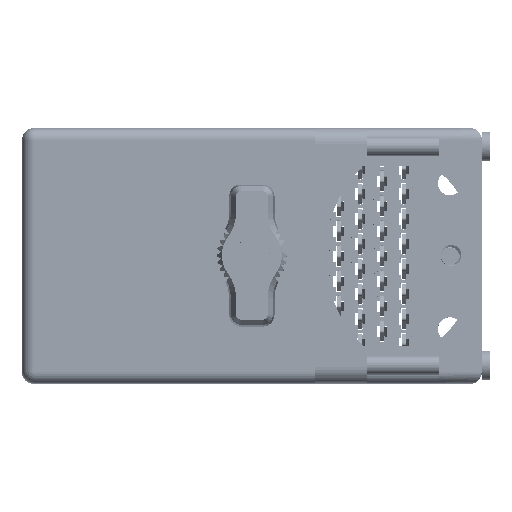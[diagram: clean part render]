
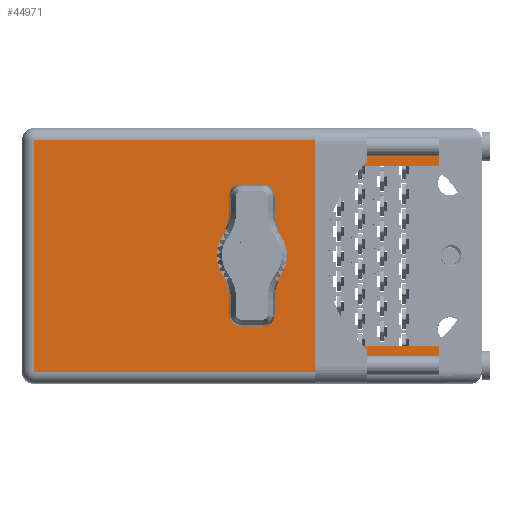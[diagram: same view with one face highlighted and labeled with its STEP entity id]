
A CAD part, top view. The second image highlights one B-rep face of the part: STEP entity #44971.
In plain terms, the highlighted face is planar.
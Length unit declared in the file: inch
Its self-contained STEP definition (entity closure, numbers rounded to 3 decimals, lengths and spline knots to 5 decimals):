
#1063 = DIRECTION ( 'NONE',  ( 0., 1., 0. ) ) ;
#3258 = AXIS2_PLACEMENT_3D ( 'NONE', #57674, #67712, #58091 ) ;
#4611 = CARTESIAN_POINT ( 'NONE',  ( 2.499, 2.03, -0.07 ) ) ;
#10472 = EDGE_CURVE ( 'NONE', #17656, #46219, #93250, .T. ) ;
#11401 = CARTESIAN_POINT ( 'NONE',  ( 1.3775, 2.03, -0.935 ) ) ;
#11614 = CARTESIAN_POINT ( 'NONE',  ( 2.499, 2.03, -1.305 ) ) ;
#12439 = ORIENTED_EDGE ( 'NONE', *, *, #10472, .F. ) ;
#12688 = CARTESIAN_POINT ( 'NONE',  ( 1.785, 2.03, -1.305 ) ) ;
#13154 = LINE ( 'NONE', #12688, #102062 ) ;
#13281 = LINE ( 'NONE', #101350, #80673 ) ;
#14627 = LINE ( 'NONE', #4611, #59185 ) ;
#15113 = CARTESIAN_POINT ( 'NONE',  ( 1.3775, 2.03, -0.595 ) ) ;
#15484 = VECTOR ( 'NONE', #58173, 39.37008 ) ;
#16676 = CIRCLE ( 'NONE', #3258, 0.17 ) ;
#17132 = EDGE_CURVE ( 'NONE', #26640, #64895, #16676, .T. ) ;
#17282 = VECTOR ( 'NONE', #108263, 39.37008 ) ;
#17656 = VERTEX_POINT ( 'NONE', #29456 ) ;
#19880 = ORIENTED_EDGE ( 'NONE', *, *, #88196, .T. ) ;
#20483 = EDGE_CURVE ( 'NONE', #95439, #37082, #14627, .T. ) ;
#22983 = VERTEX_POINT ( 'NONE', #118377 ) ;
#26640 = VERTEX_POINT ( 'NONE', #15113 ) ;
#27011 = VERTEX_POINT ( 'NONE', #96751 ) ;
#29456 = CARTESIAN_POINT ( 'NONE',  ( 2.499, 2.03, -1.46 ) ) ;
#30545 = CARTESIAN_POINT ( 'NONE',  ( 2.499, 2.03, -1.53 ) ) ;
#31002 = ORIENTED_EDGE ( 'NONE', *, *, #17132, .F. ) ;
#33151 = ORIENTED_EDGE ( 'NONE', *, *, #20483, .T. ) ;
#34636 = CARTESIAN_POINT ( 'NONE',  ( 2.499, 2.03, -0.225 ) ) ;
#35036 = DIRECTION ( 'NONE',  ( -1., 0., 0. ) ) ;
#37082 = VERTEX_POINT ( 'NONE', #37415 ) ;
#37415 = CARTESIAN_POINT ( 'NONE',  ( 2.499, 2.03, -0.07 ) ) ;
#39052 = CARTESIAN_POINT ( 'NONE',  ( 1.3775, 2.03, -0.765 ) ) ;
#39896 = DIRECTION ( 'NONE',  ( 1., 0., 0. ) ) ;
#40355 = DIRECTION ( 'NONE',  ( 0., 0., -1. ) ) ;
#41054 = CARTESIAN_POINT ( 'NONE',  ( 0., 2.03, -1.46 ) ) ;
#41513 = DIRECTION ( 'NONE',  ( 1., 0., 0. ) ) ;
#42954 = VECTOR ( 'NONE', #39896, 39.37008 ) ;
#44971 = ADVANCED_FACE ( 'NONE', ( #88420, #97085 ), #94040, .T. ) ;
#46219 = VERTEX_POINT ( 'NONE', #11614 ) ;
#48017 = VERTEX_POINT ( 'NONE', #99673 ) ;
#54576 = LINE ( 'NONE', #58379, #42954 ) ;
#56519 = ORIENTED_EDGE ( 'NONE', *, *, #62419, .F. ) ;
#57674 = CARTESIAN_POINT ( 'NONE',  ( 1.3775, 2.03, -0.765 ) ) ;
#58091 = DIRECTION ( 'NONE',  ( 0., 0., 1. ) ) ;
#58173 = DIRECTION ( 'NONE',  ( 0., 0., 1. ) ) ;
#58379 = CARTESIAN_POINT ( 'NONE',  ( 2.499, 2.03, -1.305 ) ) ;
#59185 = VECTOR ( 'NONE', #41513, 39.37008 ) ;
#60343 = ORIENTED_EDGE ( 'NONE', *, *, #95100, .T. ) ;
#62419 = EDGE_CURVE ( 'NONE', #27011, #37082, #64269, .T. ) ;
#63584 = EDGE_LOOP ( 'NONE', ( #31002, #70341 ) ) ;
#63611 = ORIENTED_EDGE ( 'NONE', *, *, #115660, .T. ) ;
#64269 = LINE ( 'NONE', #68181, #15484 ) ;
#64895 = VERTEX_POINT ( 'NONE', #11401 ) ;
#66310 = VERTEX_POINT ( 'NONE', #114602 ) ;
#66632 = CIRCLE ( 'NONE', #73821, 0.17 ) ;
#67712 = DIRECTION ( 'NONE',  ( 0., 1., 0. ) ) ;
#68181 = CARTESIAN_POINT ( 'NONE',  ( 2.499, 2.03, -1.53 ) ) ;
#69373 = EDGE_CURVE ( 'NONE', #66310, #48017, #13154, .T. ) ;
#70341 = ORIENTED_EDGE ( 'NONE', *, *, #89043, .F. ) ;
#71436 = AXIS2_PLACEMENT_3D ( 'NONE', #83630, #1063, #92445 ) ;
#72680 = CARTESIAN_POINT ( 'NONE',  ( 0.07, 2.03, -0.07 ) ) ;
#73821 = AXIS2_PLACEMENT_3D ( 'NONE', #39052, #111651, #74724 ) ;
#74724 = DIRECTION ( 'NONE',  ( 0., 0., 1. ) ) ;
#75353 = ORIENTED_EDGE ( 'NONE', *, *, #69373, .T. ) ;
#75983 = VECTOR ( 'NONE', #105598, 39.37008 ) ;
#80673 = VECTOR ( 'NONE', #109787, 39.37008 ) ;
#83630 = CARTESIAN_POINT ( 'NONE',  ( 0., 2.03, -1.53 ) ) ;
#88196 = EDGE_CURVE ( 'NONE', #22983, #95439, #13281, .T. ) ;
#88420 = FACE_OUTER_BOUND ( 'NONE', #101440, .T. ) ;
#89043 = EDGE_CURVE ( 'NONE', #64895, #26640, #66632, .T. ) ;
#91278 = VECTOR ( 'NONE', #35036, 39.37008 ) ;
#92445 = DIRECTION ( 'NONE',  ( 0., 0., 1. ) ) ;
#93250 = LINE ( 'NONE', #30545, #17282 ) ;
#94040 = PLANE ( 'NONE',  #71436 ) ;
#95100 = EDGE_CURVE ( 'NONE', #48017, #46219, #54576, .T. ) ;
#95439 = VERTEX_POINT ( 'NONE', #72680 ) ;
#96751 = CARTESIAN_POINT ( 'NONE',  ( 2.499, 2.03, -0.225 ) ) ;
#97085 = FACE_BOUND ( 'NONE', #63584, .T. ) ;
#97536 = ORIENTED_EDGE ( 'NONE', *, *, #117523, .T. ) ;
#99673 = CARTESIAN_POINT ( 'NONE',  ( 1.785, 2.03, -1.305 ) ) ;
#101350 = CARTESIAN_POINT ( 'NONE',  ( 0.07, 2.03, -1.53 ) ) ;
#101440 = EDGE_LOOP ( 'NONE', ( #19880, #33151, #56519, #97536, #75353, #60343, #12439, #63611 ) ) ;
#102062 = VECTOR ( 'NONE', #40355, 39.37008 ) ;
#105598 = DIRECTION ( 'NONE',  ( -1., 0., 0. ) ) ;
#108263 = DIRECTION ( 'NONE',  ( 0., 0., 1. ) ) ;
#109044 = LINE ( 'NONE', #41054, #75983 ) ;
#109787 = DIRECTION ( 'NONE',  ( 0., 0., 1. ) ) ;
#111651 = DIRECTION ( 'NONE',  ( 0., 1., 0. ) ) ;
#114602 = CARTESIAN_POINT ( 'NONE',  ( 1.785, 2.03, -0.225 ) ) ;
#115660 = EDGE_CURVE ( 'NONE', #17656, #22983, #109044, .T. ) ;
#115734 = LINE ( 'NONE', #34636, #91278 ) ;
#117523 = EDGE_CURVE ( 'NONE', #27011, #66310, #115734, .T. ) ;
#118377 = CARTESIAN_POINT ( 'NONE',  ( 0.07, 2.03, -1.46 ) ) ;
